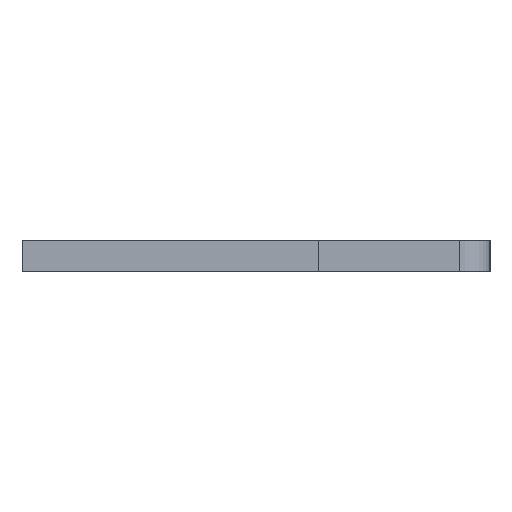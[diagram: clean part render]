
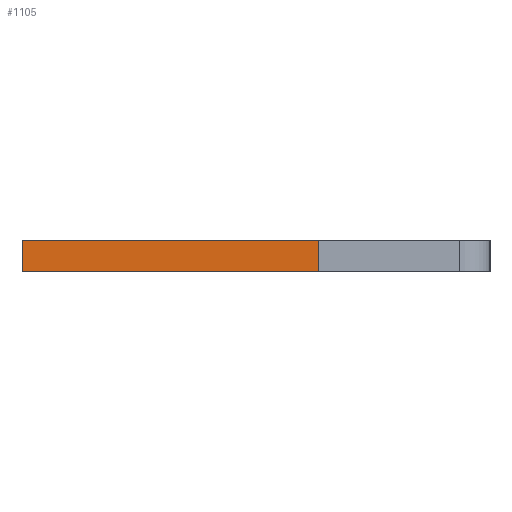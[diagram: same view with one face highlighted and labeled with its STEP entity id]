
A CAD part, left-side view. The second image highlights one B-rep face of the part: STEP entity #1105.
In plain terms, the highlighted face is planar.
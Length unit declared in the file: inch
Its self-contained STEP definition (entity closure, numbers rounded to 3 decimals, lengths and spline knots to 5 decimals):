
#65 = AXIS2_PLACEMENT_3D ( 'NONE', #474, #115, #1349 ) ;
#115 = DIRECTION ( 'NONE',  ( 0., 0., 1. ) ) ;
#150 = EDGE_CURVE ( 'NONE', #885, #905, #862, .T. ) ;
#202 = VECTOR ( 'NONE', #1109, 39.37008 ) ;
#217 = FACE_OUTER_BOUND ( 'NONE', #1246, .T. ) ;
#322 = EDGE_CURVE ( 'NONE', #905, #1100, #388, .T. ) ;
#367 = CARTESIAN_POINT ( 'NONE',  ( -0.01, 0.15, -0.04 ) ) ;
#388 = LINE ( 'NONE', #1010, #458 ) ;
#418 = DIRECTION ( 'NONE',  ( -1., 0., 0. ) ) ;
#419 = ORIENTED_EDGE ( 'NONE', *, *, #609, .F. ) ;
#458 = VECTOR ( 'NONE', #1372, 39.37008 ) ;
#474 = CARTESIAN_POINT ( 'NONE',  ( 0.01, 0.15, -0.04 ) ) ;
#548 = ORIENTED_EDGE ( 'NONE', *, *, #150, .T. ) ;
#571 = CARTESIAN_POINT ( 'NONE',  ( -0.01, -0.04, -0.04 ) ) ;
#592 = CARTESIAN_POINT ( 'NONE',  ( 0.01, 0.15, -0.04 ) ) ;
#608 = VECTOR ( 'NONE', #418, 39.37008 ) ;
#609 = EDGE_CURVE ( 'NONE', #1004, #1100, #650, .T. ) ;
#636 = ORIENTED_EDGE ( 'NONE', *, *, #1472, .F. ) ;
#650 = LINE ( 'NONE', #1036, #608 ) ;
#822 = PLANE ( 'NONE',  #65 ) ;
#862 = LINE ( 'NONE', #978, #202 ) ;
#878 = VECTOR ( 'NONE', #1281, 39.37008 ) ;
#885 = VERTEX_POINT ( 'NONE', #1203 ) ;
#905 = VERTEX_POINT ( 'NONE', #571 ) ;
#978 = CARTESIAN_POINT ( 'NONE',  ( 0.01, -0.04, -0.04 ) ) ;
#1004 = VERTEX_POINT ( 'NONE', #592 ) ;
#1010 = CARTESIAN_POINT ( 'NONE',  ( -0.01, 0.15, -0.04 ) ) ;
#1036 = CARTESIAN_POINT ( 'NONE',  ( 0.01, 0.15, -0.04 ) ) ;
#1100 = VERTEX_POINT ( 'NONE', #367 ) ;
#1105 = ADVANCED_FACE ( 'NONE', ( #217 ), #822, .F. ) ;
#1109 = DIRECTION ( 'NONE',  ( -1., 0., 0. ) ) ;
#1167 = CARTESIAN_POINT ( 'NONE',  ( 0.01, 0.15, -0.04 ) ) ;
#1203 = CARTESIAN_POINT ( 'NONE',  ( 0.01, -0.04, -0.04 ) ) ;
#1246 = EDGE_LOOP ( 'NONE', ( #1532, #419, #636, #548 ) ) ;
#1281 = DIRECTION ( 'NONE',  ( 0., 1., 0. ) ) ;
#1322 = LINE ( 'NONE', #1167, #878 ) ;
#1349 = DIRECTION ( 'NONE',  ( 1., 0., 0. ) ) ;
#1372 = DIRECTION ( 'NONE',  ( 0., 1., 0. ) ) ;
#1472 = EDGE_CURVE ( 'NONE', #885, #1004, #1322, .T. ) ;
#1532 = ORIENTED_EDGE ( 'NONE', *, *, #322, .T. ) ;
